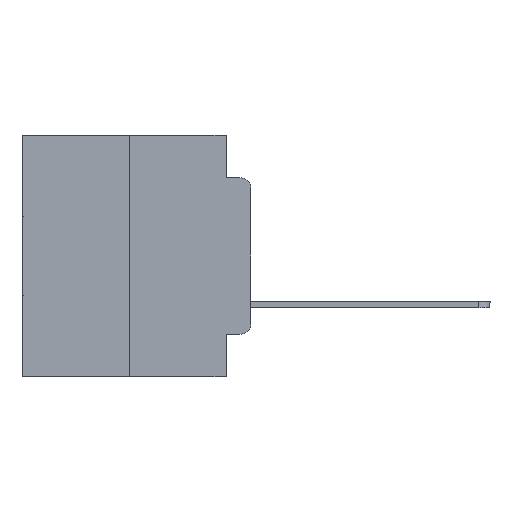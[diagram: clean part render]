
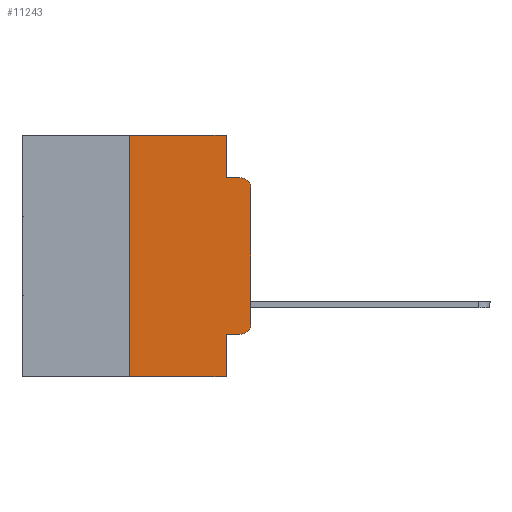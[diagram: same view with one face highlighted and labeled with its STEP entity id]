
A CAD part, left-side view. The second image highlights one B-rep face of the part: STEP entity #11243.
In plain terms, the highlighted planar face has unit normal (-1, 0, 0).
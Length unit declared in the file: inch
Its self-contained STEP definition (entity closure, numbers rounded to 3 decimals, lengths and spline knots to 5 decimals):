
#1049 = LINE ( 'NONE', #10436, #25166 ) ;
#1311 = VERTEX_POINT ( 'NONE', #24437 ) ;
#1351 = VECTOR ( 'NONE', #13100, 39.37008 ) ;
#1830 = EDGE_CURVE ( 'NONE', #20528, #25834, #15486, .T. ) ;
#1967 = VECTOR ( 'NONE', #21785, 39.37008 ) ;
#2415 = DIRECTION ( 'NONE',  ( 0., -1., 0. ) ) ;
#2571 = CARTESIAN_POINT ( 'NONE',  ( 0., 0.051, 0. ) ) ;
#2707 = LINE ( 'NONE', #11786, #26800 ) ;
#3157 = VERTEX_POINT ( 'NONE', #2571 ) ;
#3640 = CARTESIAN_POINT ( 'NONE',  ( 0., 0.25, 0. ) ) ;
#3643 = CARTESIAN_POINT ( 'NONE',  ( 0., 0.051, -0.4115 ) ) ;
#4027 = CARTESIAN_POINT ( 'NONE',  ( 0., 0., 0. ) ) ;
#4034 = VERTEX_POINT ( 'NONE', #13073 ) ;
#4186 = EDGE_CURVE ( 'NONE', #3157, #1311, #16616, .T. ) ;
#4506 = LINE ( 'NONE', #5097, #15471 ) ;
#4795 = ORIENTED_EDGE ( 'NONE', *, *, #7069, .T. ) ;
#4892 = CARTESIAN_POINT ( 'NONE',  ( 0., 0.051, 0. ) ) ;
#5097 = CARTESIAN_POINT ( 'NONE',  ( 0., 0.473, -0.5 ) ) ;
#5549 = ORIENTED_EDGE ( 'NONE', *, *, #26112, .F. ) ;
#5913 = CARTESIAN_POINT ( 'NONE',  ( 0., 0.051, 0. ) ) ;
#6066 = EDGE_CURVE ( 'NONE', #22948, #20777, #24009, .T. ) ;
#7069 = EDGE_CURVE ( 'NONE', #7197, #20528, #28964, .T. ) ;
#7197 = VERTEX_POINT ( 'NONE', #11751 ) ;
#7328 = ORIENTED_EDGE ( 'NONE', *, *, #6066, .T. ) ;
#7562 = ORIENTED_EDGE ( 'NONE', *, *, #1830, .T. ) ;
#7817 = VERTEX_POINT ( 'NONE', #18038 ) ;
#8126 = EDGE_CURVE ( 'NONE', #7817, #12390, #1049, .T. ) ;
#8472 = EDGE_LOOP ( 'NONE', ( #4795, #7562, #24958, #12362, #8488, #14326, #9820, #5549, #7328, #21875 ) ) ;
#8488 = ORIENTED_EDGE ( 'NONE', *, *, #16661, .F. ) ;
#8837 = DIRECTION ( 'NONE',  ( 1., 0., 0. ) ) ;
#8871 = AXIS2_PLACEMENT_3D ( 'NONE', #15214, #24269, #10757 ) ;
#9820 = ORIENTED_EDGE ( 'NONE', *, *, #16721, .T. ) ;
#9821 = CARTESIAN_POINT ( 'NONE',  ( 0., 0., -0.1085 ) ) ;
#10436 = CARTESIAN_POINT ( 'NONE',  ( 0., 0.25, 0. ) ) ;
#10757 = DIRECTION ( 'NONE',  ( 0., 0., -1. ) ) ;
#11243 = ADVANCED_FACE ( 'NONE', ( #18037 ), #11511, .F. ) ;
#11511 = PLANE ( 'NONE',  #29010 ) ;
#11593 = CARTESIAN_POINT ( 'NONE',  ( 0., 0.02, -0.0885 ) ) ;
#11751 = CARTESIAN_POINT ( 'NONE',  ( 0., 0., -0.3915 ) ) ;
#11786 = CARTESIAN_POINT ( 'NONE',  ( 0., 0.473, 0. ) ) ;
#11961 = CARTESIAN_POINT ( 'NONE',  ( 0., 0.02, -0.4115 ) ) ;
#12362 = ORIENTED_EDGE ( 'NONE', *, *, #4186, .F. ) ;
#12390 = VERTEX_POINT ( 'NONE', #3640 ) ;
#12644 = VECTOR ( 'NONE', #23146, 39.37008 ) ;
#12812 = DIRECTION ( 'NONE',  ( 0., 0., 1. ) ) ;
#13022 = DIRECTION ( 'NONE',  ( 0., -1., 0. ) ) ;
#13073 = CARTESIAN_POINT ( 'NONE',  ( 0., 0.051, -0.5 ) ) ;
#13100 = DIRECTION ( 'NONE',  ( 0., 0., 1. ) ) ;
#13437 = CARTESIAN_POINT ( 'NONE',  ( 0., 0.473, 0. ) ) ;
#13696 = DIRECTION ( 'NONE',  ( 0., 0., -1. ) ) ;
#14129 = CARTESIAN_POINT ( 'NONE',  ( 0., 0.02, -0.3915 ) ) ;
#14326 = ORIENTED_EDGE ( 'NONE', *, *, #8126, .F. ) ;
#14801 = LINE ( 'NONE', #24145, #22410 ) ;
#15214 = CARTESIAN_POINT ( 'NONE',  ( 0., 0.02, -0.1085 ) ) ;
#15471 = VECTOR ( 'NONE', #16238, 39.37008 ) ;
#15486 = CIRCLE ( 'NONE', #8871, 0.02 ) ;
#16238 = DIRECTION ( 'NONE',  ( 0., -1., 0. ) ) ;
#16616 = LINE ( 'NONE', #4892, #12644 ) ;
#16661 = EDGE_CURVE ( 'NONE', #12390, #3157, #2707, .T. ) ;
#16721 = EDGE_CURVE ( 'NONE', #7817, #4034, #4506, .T. ) ;
#18037 = FACE_OUTER_BOUND ( 'NONE', #8472, .T. ) ;
#18038 = CARTESIAN_POINT ( 'NONE',  ( 0., 0.25, -0.5 ) ) ;
#18380 = EDGE_CURVE ( 'NONE', #20777, #7197, #24457, .T. ) ;
#20528 = VERTEX_POINT ( 'NONE', #9821 ) ;
#20674 = AXIS2_PLACEMENT_3D ( 'NONE', #14129, #24954, #13696 ) ;
#20777 = VERTEX_POINT ( 'NONE', #11961 ) ;
#21785 = DIRECTION ( 'NONE',  ( 0., 0., -1. ) ) ;
#21875 = ORIENTED_EDGE ( 'NONE', *, *, #18380, .T. ) ;
#22410 = VECTOR ( 'NONE', #26215, 39.37008 ) ;
#22948 = VERTEX_POINT ( 'NONE', #23177 ) ;
#23146 = DIRECTION ( 'NONE',  ( 0., 0., -1. ) ) ;
#23177 = CARTESIAN_POINT ( 'NONE',  ( 0., 0.051, -0.4115 ) ) ;
#24009 = LINE ( 'NONE', #3643, #24794 ) ;
#24145 = CARTESIAN_POINT ( 'NONE',  ( 0., 0.051, -0.0885 ) ) ;
#24269 = DIRECTION ( 'NONE',  ( -1., 0., 0. ) ) ;
#24437 = CARTESIAN_POINT ( 'NONE',  ( 0., 0.051, -0.0885 ) ) ;
#24457 = CIRCLE ( 'NONE', #20674, 0.02 ) ;
#24794 = VECTOR ( 'NONE', #13022, 39.37008 ) ;
#24954 = DIRECTION ( 'NONE',  ( -1., 0., 0. ) ) ;
#24958 = ORIENTED_EDGE ( 'NONE', *, *, #26694, .F. ) ;
#25166 = VECTOR ( 'NONE', #12812, 39.37008 ) ;
#25834 = VERTEX_POINT ( 'NONE', #11593 ) ;
#26112 = EDGE_CURVE ( 'NONE', #22948, #4034, #26537, .T. ) ;
#26215 = DIRECTION ( 'NONE',  ( 0., -1., 0. ) ) ;
#26537 = LINE ( 'NONE', #5913, #1967 ) ;
#26694 = EDGE_CURVE ( 'NONE', #1311, #25834, #14801, .T. ) ;
#26800 = VECTOR ( 'NONE', #2415, 39.37008 ) ;
#26928 = DIRECTION ( 'NONE',  ( 0., 0., -1. ) ) ;
#28964 = LINE ( 'NONE', #4027, #1351 ) ;
#29010 = AXIS2_PLACEMENT_3D ( 'NONE', #13437, #8837, #26928 ) ;
